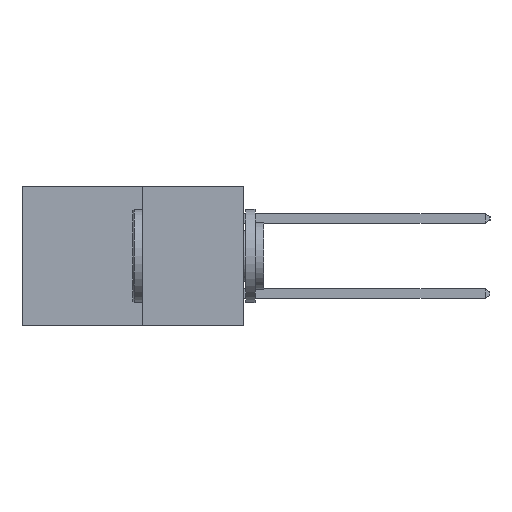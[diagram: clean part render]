
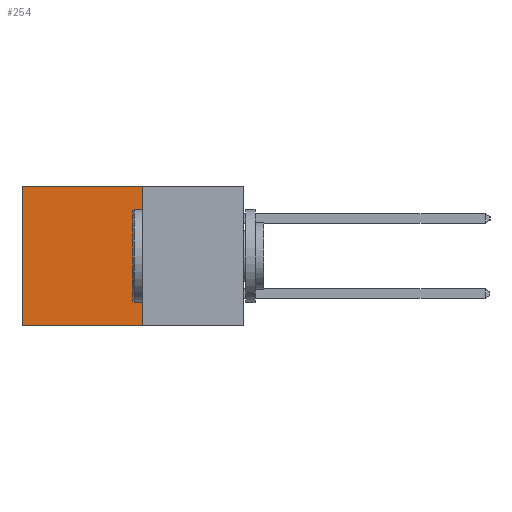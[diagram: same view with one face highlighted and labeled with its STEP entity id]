
A CAD part, left-side view. The second image highlights one B-rep face of the part: STEP entity #254.
In plain terms, the highlighted planar face has unit normal (-1, 0, 0).
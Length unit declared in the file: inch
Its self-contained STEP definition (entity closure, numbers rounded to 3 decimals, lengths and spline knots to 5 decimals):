
#254 = ADVANCED_FACE ( 'NONE', ( #25401 ), #23581, .F. ) ;
#1381 = CARTESIAN_POINT ( 'NONE',  ( 0.277, 0.27, -0.37 ) ) ;
#1668 = AXIS2_PLACEMENT_3D ( 'NONE', #23710, #8513, #18604 ) ;
#1814 = CARTESIAN_POINT ( 'NONE',  ( 0.277, 0.27, 0. ) ) ;
#2566 = CARTESIAN_POINT ( 'NONE',  ( 0.277, 0.27, -0.37 ) ) ;
#2619 = EDGE_CURVE ( 'NONE', #4574, #5560, #10456, .T. ) ;
#3959 = CARTESIAN_POINT ( 'NONE',  ( 0.277, 0.59, 0. ) ) ;
#4574 = VERTEX_POINT ( 'NONE', #3959 ) ;
#5439 = ORIENTED_EDGE ( 'NONE', *, *, #2619, .T. ) ;
#5560 = VERTEX_POINT ( 'NONE', #25844 ) ;
#5683 = EDGE_CURVE ( 'NONE', #25432, #5560, #15655, .T. ) ;
#8301 = CARTESIAN_POINT ( 'NONE',  ( 0.277, 0.27, 0. ) ) ;
#8513 = DIRECTION ( 'NONE',  ( 1., 0., 0. ) ) ;
#9624 = VECTOR ( 'NONE', #19580, 39.37008 ) ;
#10298 = VERTEX_POINT ( 'NONE', #1814 ) ;
#10456 = LINE ( 'NONE', #28120, #23199 ) ;
#13088 = CARTESIAN_POINT ( 'NONE',  ( 0.277, 0.27, -0.37 ) ) ;
#15655 = LINE ( 'NONE', #1381, #9624 ) ;
#16273 = DIRECTION ( 'NONE',  ( 0., 0., -1. ) ) ;
#17193 = EDGE_LOOP ( 'NONE', ( #5439, #18341, #21804, #24949 ) ) ;
#18341 = ORIENTED_EDGE ( 'NONE', *, *, #5683, .F. ) ;
#18604 = DIRECTION ( 'NONE',  ( 0., 0., -1. ) ) ;
#19059 = VECTOR ( 'NONE', #16273, 39.37008 ) ;
#19209 = VECTOR ( 'NONE', #28493, 39.37008 ) ;
#19580 = DIRECTION ( 'NONE',  ( 0., 1., 0. ) ) ;
#21804 = ORIENTED_EDGE ( 'NONE', *, *, #24581, .F. ) ;
#23199 = VECTOR ( 'NONE', #26728, 39.37008 ) ;
#23581 = PLANE ( 'NONE',  #1668 ) ;
#23710 = CARTESIAN_POINT ( 'NONE',  ( 0.277, 0.27, -0.37 ) ) ;
#24581 = EDGE_CURVE ( 'NONE', #10298, #25432, #24924, .T. ) ;
#24924 = LINE ( 'NONE', #2566, #19059 ) ;
#24949 = ORIENTED_EDGE ( 'NONE', *, *, #28506, .T. ) ;
#25401 = FACE_OUTER_BOUND ( 'NONE', #17193, .T. ) ;
#25432 = VERTEX_POINT ( 'NONE', #13088 ) ;
#25760 = LINE ( 'NONE', #8301, #19209 ) ;
#25844 = CARTESIAN_POINT ( 'NONE',  ( 0.277, 0.59, -0.37 ) ) ;
#26728 = DIRECTION ( 'NONE',  ( 0., 0., -1. ) ) ;
#28120 = CARTESIAN_POINT ( 'NONE',  ( 0.277, 0.59, -0.37 ) ) ;
#28493 = DIRECTION ( 'NONE',  ( 0., 1., 0. ) ) ;
#28506 = EDGE_CURVE ( 'NONE', #10298, #4574, #25760, .T. ) ;
